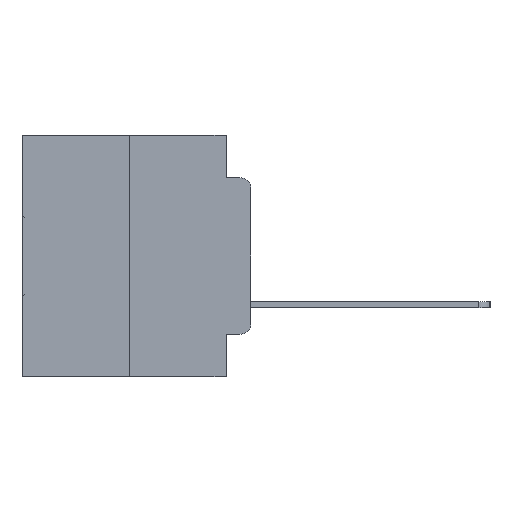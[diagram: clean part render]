
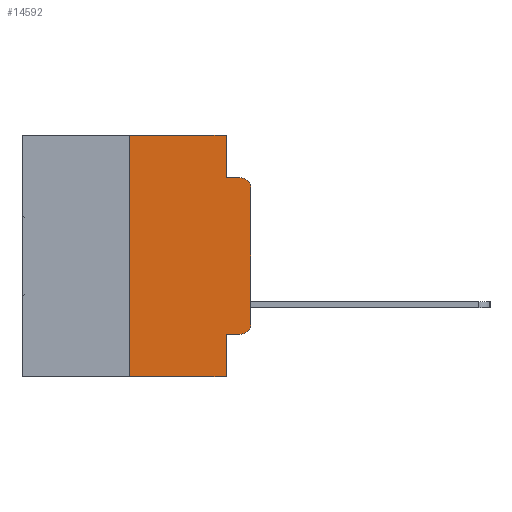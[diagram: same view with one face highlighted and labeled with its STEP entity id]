
A CAD part, left-side view. The second image highlights one B-rep face of the part: STEP entity #14592.
In plain terms, the highlighted planar face has unit normal (-1, 0, 0).
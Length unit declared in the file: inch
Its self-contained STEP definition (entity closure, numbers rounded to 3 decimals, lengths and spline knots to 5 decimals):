
#105 = CARTESIAN_POINT ( 'NONE',  ( 0., 0.02, -0.4115 ) ) ;
#201 = VERTEX_POINT ( 'NONE', #11270 ) ;
#674 = ORIENTED_EDGE ( 'NONE', *, *, #29700, .T. ) ;
#1272 = PLANE ( 'NONE',  #22409 ) ;
#1974 = ORIENTED_EDGE ( 'NONE', *, *, #28948, .F. ) ;
#2219 = VERTEX_POINT ( 'NONE', #6263 ) ;
#2460 = ORIENTED_EDGE ( 'NONE', *, *, #30122, .T. ) ;
#2467 = CARTESIAN_POINT ( 'NONE',  ( 0., 0.051, -0.0885 ) ) ;
#2510 = LINE ( 'NONE', #19450, #13884 ) ;
#2623 = LINE ( 'NONE', #24956, #27091 ) ;
#2777 = CARTESIAN_POINT ( 'NONE',  ( 0., 0., -0.3915 ) ) ;
#3858 = DIRECTION ( 'NONE',  ( 1., 0., 0. ) ) ;
#6263 = CARTESIAN_POINT ( 'NONE',  ( 0., 0.25, -0.5 ) ) ;
#6380 = DIRECTION ( 'NONE',  ( 0., -1., 0. ) ) ;
#6980 = VERTEX_POINT ( 'NONE', #17525 ) ;
#7115 = DIRECTION ( 'NONE',  ( 0., -1., 0. ) ) ;
#7720 = CARTESIAN_POINT ( 'NONE',  ( 0., 0.25, 0. ) ) ;
#7793 = DIRECTION ( 'NONE',  ( 0., 0., 1. ) ) ;
#8204 = ORIENTED_EDGE ( 'NONE', *, *, #28427, .F. ) ;
#8875 = DIRECTION ( 'NONE',  ( -1., 0., 0. ) ) ;
#9510 = ORIENTED_EDGE ( 'NONE', *, *, #16214, .F. ) ;
#9599 = LINE ( 'NONE', #27588, #26734 ) ;
#10283 = LINE ( 'NONE', #23553, #27366 ) ;
#11133 = CARTESIAN_POINT ( 'NONE',  ( 0., 0.473, 0. ) ) ;
#11270 = CARTESIAN_POINT ( 'NONE',  ( 0., 0.25, 0. ) ) ;
#11486 = FACE_OUTER_BOUND ( 'NONE', #28159, .T. ) ;
#11619 = ORIENTED_EDGE ( 'NONE', *, *, #26200, .T. ) ;
#12055 = VERTEX_POINT ( 'NONE', #26151 ) ;
#12353 = CARTESIAN_POINT ( 'NONE',  ( 0., 0.02, -0.3915 ) ) ;
#12490 = DIRECTION ( 'NONE',  ( 0., 0., 1. ) ) ;
#13126 = DIRECTION ( 'NONE',  ( 0., -1., 0. ) ) ;
#13531 = VECTOR ( 'NONE', #13126, 39.37008 ) ;
#13884 = VECTOR ( 'NONE', #7793, 39.37008 ) ;
#14255 = AXIS2_PLACEMENT_3D ( 'NONE', #22899, #8875, #25232 ) ;
#14293 = VERTEX_POINT ( 'NONE', #2777 ) ;
#14300 = CIRCLE ( 'NONE', #18437, 0.02 ) ;
#14592 = ADVANCED_FACE ( 'NONE', ( #11486 ), #1272, .F. ) ;
#14693 = DIRECTION ( 'NONE',  ( 0., 0., -1. ) ) ;
#15765 = ORIENTED_EDGE ( 'NONE', *, *, #28184, .F. ) ;
#16214 = EDGE_CURVE ( 'NONE', #201, #20519, #10283, .T. ) ;
#16336 = ORIENTED_EDGE ( 'NONE', *, *, #26581, .F. ) ;
#16478 = VECTOR ( 'NONE', #12490, 39.37008 ) ;
#16686 = ORIENTED_EDGE ( 'NONE', *, *, #25839, .T. ) ;
#16823 = VECTOR ( 'NONE', #20939, 39.37008 ) ;
#17525 = CARTESIAN_POINT ( 'NONE',  ( 0., 0.051, -0.4115 ) ) ;
#17778 = CARTESIAN_POINT ( 'NONE',  ( 0., 0.051, -0.0885 ) ) ;
#17926 = LINE ( 'NONE', #29062, #18650 ) ;
#17968 = DIRECTION ( 'NONE',  ( 0., -1., 0. ) ) ;
#18437 = AXIS2_PLACEMENT_3D ( 'NONE', #12353, #28581, #14693 ) ;
#18650 = VECTOR ( 'NONE', #22230, 39.37008 ) ;
#18960 = LINE ( 'NONE', #17778, #13531 ) ;
#19450 = CARTESIAN_POINT ( 'NONE',  ( 0., 0., 0. ) ) ;
#20434 = DIRECTION ( 'NONE',  ( 0., 0., -1. ) ) ;
#20519 = VERTEX_POINT ( 'NONE', #22945 ) ;
#20836 = CARTESIAN_POINT ( 'NONE',  ( 0., 0.051, 0. ) ) ;
#20939 = DIRECTION ( 'NONE',  ( 0., 0., -1. ) ) ;
#21167 = LINE ( 'NONE', #7720, #16478 ) ;
#21643 = VERTEX_POINT ( 'NONE', #29780 ) ;
#22045 = EDGE_CURVE ( 'NONE', #2219, #12055, #2623, .T. ) ;
#22230 = DIRECTION ( 'NONE',  ( 0., 0., -1. ) ) ;
#22409 = AXIS2_PLACEMENT_3D ( 'NONE', #11133, #3858, #20434 ) ;
#22899 = CARTESIAN_POINT ( 'NONE',  ( 0., 0.02, -0.1085 ) ) ;
#22945 = CARTESIAN_POINT ( 'NONE',  ( 0., 0.051, 0. ) ) ;
#23040 = LINE ( 'NONE', #20836, #16823 ) ;
#23553 = CARTESIAN_POINT ( 'NONE',  ( 0., 0.473, 0. ) ) ;
#24956 = CARTESIAN_POINT ( 'NONE',  ( 0., 0.473, -0.5 ) ) ;
#25232 = DIRECTION ( 'NONE',  ( 0., 0., -1. ) ) ;
#25293 = VERTEX_POINT ( 'NONE', #2467 ) ;
#25533 = CIRCLE ( 'NONE', #14255, 0.02 ) ;
#25795 = ORIENTED_EDGE ( 'NONE', *, *, #22045, .T. ) ;
#25839 = EDGE_CURVE ( 'NONE', #28155, #14293, #14300, .T. ) ;
#26151 = CARTESIAN_POINT ( 'NONE',  ( 0., 0.051, -0.5 ) ) ;
#26200 = EDGE_CURVE ( 'NONE', #6980, #28155, #9599, .T. ) ;
#26355 = CARTESIAN_POINT ( 'NONE',  ( 0., 0.02, -0.0885 ) ) ;
#26581 = EDGE_CURVE ( 'NONE', #6980, #12055, #17926, .T. ) ;
#26734 = VECTOR ( 'NONE', #6380, 39.37008 ) ;
#27091 = VECTOR ( 'NONE', #17968, 39.37008 ) ;
#27366 = VECTOR ( 'NONE', #7115, 39.37008 ) ;
#27588 = CARTESIAN_POINT ( 'NONE',  ( 0., 0.051, -0.4115 ) ) ;
#28119 = VERTEX_POINT ( 'NONE', #26355 ) ;
#28155 = VERTEX_POINT ( 'NONE', #105 ) ;
#28159 = EDGE_LOOP ( 'NONE', ( #2460, #674, #1974, #8204, #9510, #15765, #25795, #16336, #11619, #16686 ) ) ;
#28184 = EDGE_CURVE ( 'NONE', #2219, #201, #21167, .T. ) ;
#28427 = EDGE_CURVE ( 'NONE', #20519, #25293, #23040, .T. ) ;
#28581 = DIRECTION ( 'NONE',  ( -1., 0., 0. ) ) ;
#28948 = EDGE_CURVE ( 'NONE', #25293, #28119, #18960, .T. ) ;
#29062 = CARTESIAN_POINT ( 'NONE',  ( 0., 0.051, 0. ) ) ;
#29700 = EDGE_CURVE ( 'NONE', #21643, #28119, #25533, .T. ) ;
#29780 = CARTESIAN_POINT ( 'NONE',  ( 0., 0., -0.1085 ) ) ;
#30122 = EDGE_CURVE ( 'NONE', #14293, #21643, #2510, .T. ) ;
